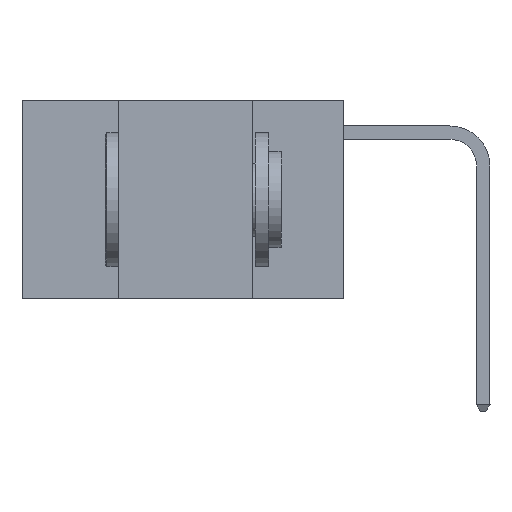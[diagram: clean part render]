
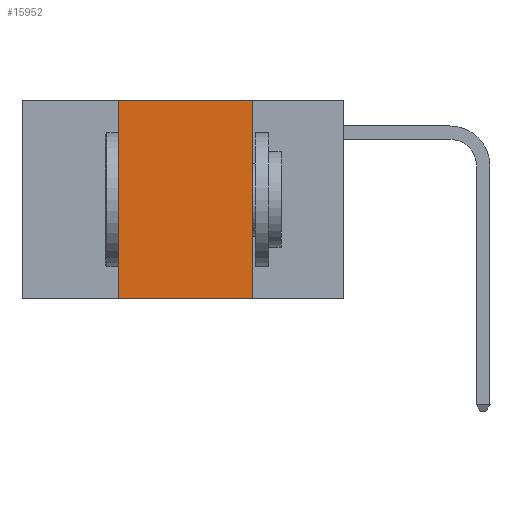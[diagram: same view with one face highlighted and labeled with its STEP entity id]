
A CAD part, left-side view. The second image highlights one B-rep face of the part: STEP entity #15952.
In plain terms, the highlighted planar face has unit normal (-1, 0, 0).
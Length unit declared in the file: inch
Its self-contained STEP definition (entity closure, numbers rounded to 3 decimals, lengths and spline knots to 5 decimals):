
#764 = EDGE_CURVE ( 'NONE', #14774, #3659, #1715, .T. ) ;
#1541 = DIRECTION ( 'NONE',  ( 1., 0., 0. ) ) ;
#1689 = CARTESIAN_POINT ( 'NONE',  ( 0., 0.42, 0. ) ) ;
#1715 = LINE ( 'NONE', #13448, #8308 ) ;
#2000 = CARTESIAN_POINT ( 'NONE',  ( 0., 0.42, 0. ) ) ;
#2069 = ORIENTED_EDGE ( 'NONE', *, *, #764, .T. ) ;
#2507 = VECTOR ( 'NONE', #5952, 39.37008 ) ;
#2850 = LINE ( 'NONE', #2000, #5922 ) ;
#3273 = VERTEX_POINT ( 'NONE', #10471 ) ;
#3407 = CARTESIAN_POINT ( 'NONE',  ( 0., 0.17, -0.37 ) ) ;
#3600 = EDGE_CURVE ( 'NONE', #7197, #3273, #16334, .T. ) ;
#3659 = VERTEX_POINT ( 'NONE', #3407 ) ;
#3871 = DIRECTION ( 'NONE',  ( 0., 0., -1. ) ) ;
#4145 = CARTESIAN_POINT ( 'NONE',  ( 0., 0.6, 0. ) ) ;
#5154 = ORIENTED_EDGE ( 'NONE', *, *, #6218, .F. ) ;
#5708 = EDGE_CURVE ( 'NONE', #3273, #3659, #10217, .T. ) ;
#5922 = VECTOR ( 'NONE', #5988, 39.37008 ) ;
#5952 = DIRECTION ( 'NONE',  ( 0., -1., 0. ) ) ;
#5988 = DIRECTION ( 'NONE',  ( 0., 0., 1. ) ) ;
#6218 = EDGE_CURVE ( 'NONE', #14774, #7197, #2850, .T. ) ;
#6770 = VECTOR ( 'NONE', #3871, 39.37008 ) ;
#7197 = VERTEX_POINT ( 'NONE', #1689 ) ;
#7915 = FACE_OUTER_BOUND ( 'NONE', #12444, .T. ) ;
#8308 = VECTOR ( 'NONE', #16842, 39.37008 ) ;
#9392 = PLANE ( 'NONE',  #10781 ) ;
#10217 = LINE ( 'NONE', #14251, #6770 ) ;
#10471 = CARTESIAN_POINT ( 'NONE',  ( 0., 0.17, 0. ) ) ;
#10731 = DIRECTION ( 'NONE',  ( 0., 0., -1. ) ) ;
#10781 = AXIS2_PLACEMENT_3D ( 'NONE', #4145, #1541, #10731 ) ;
#11144 = CARTESIAN_POINT ( 'NONE',  ( 0., 0.6, 0. ) ) ;
#12444 = EDGE_LOOP ( 'NONE', ( #14464, #15272, #5154, #2069 ) ) ;
#13448 = CARTESIAN_POINT ( 'NONE',  ( 0., 0.6, -0.37 ) ) ;
#14251 = CARTESIAN_POINT ( 'NONE',  ( 0., 0.17, 0. ) ) ;
#14464 = ORIENTED_EDGE ( 'NONE', *, *, #5708, .F. ) ;
#14774 = VERTEX_POINT ( 'NONE', #15696 ) ;
#15272 = ORIENTED_EDGE ( 'NONE', *, *, #3600, .F. ) ;
#15696 = CARTESIAN_POINT ( 'NONE',  ( 0., 0.42, -0.37 ) ) ;
#15952 = ADVANCED_FACE ( 'NONE', ( #7915 ), #9392, .F. ) ;
#16334 = LINE ( 'NONE', #11144, #2507 ) ;
#16842 = DIRECTION ( 'NONE',  ( 0., -1., 0. ) ) ;
